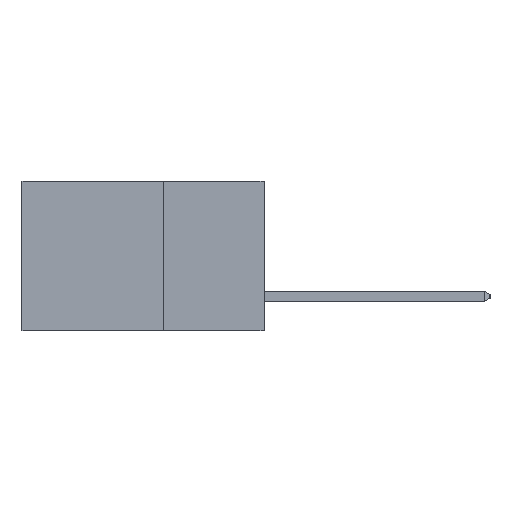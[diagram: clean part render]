
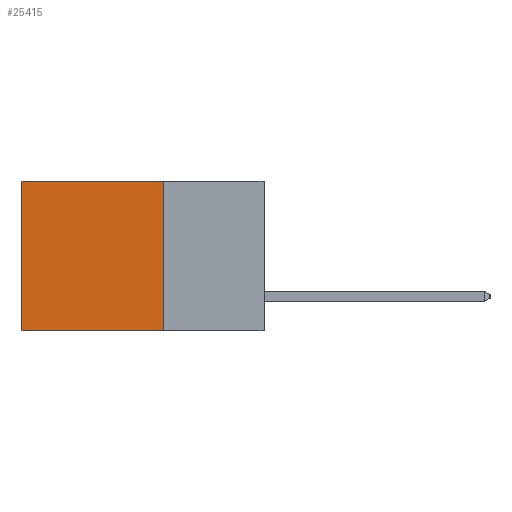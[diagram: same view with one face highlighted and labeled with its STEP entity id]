
A CAD part, left-side view. The second image highlights one B-rep face of the part: STEP entity #25415.
In plain terms, the highlighted planar face has unit normal (-1, 0, 0).
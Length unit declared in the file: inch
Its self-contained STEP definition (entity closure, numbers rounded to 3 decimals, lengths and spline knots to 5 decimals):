
#1158 = EDGE_CURVE ( 'NONE', #21931, #6660, #15601, .T. ) ;
#1533 = CARTESIAN_POINT ( 'NONE',  ( 0.298, 0.25, -0.37 ) ) ;
#1638 = LINE ( 'NONE', #1533, #12215 ) ;
#2496 = CARTESIAN_POINT ( 'NONE',  ( 0.298, 0.25, 0. ) ) ;
#2591 = DIRECTION ( 'NONE',  ( 0., 0., -1. ) ) ;
#2770 = CARTESIAN_POINT ( 'NONE',  ( 0.298, 0.25, 0. ) ) ;
#2794 = DIRECTION ( 'NONE',  ( 0., 0., -1. ) ) ;
#3395 = LINE ( 'NONE', #22034, #25294 ) ;
#3710 = DIRECTION ( 'NONE',  ( 0., 1., 0. ) ) ;
#3746 = ORIENTED_EDGE ( 'NONE', *, *, #8971, .F. ) ;
#4423 = CARTESIAN_POINT ( 'NONE',  ( 0.298, 0.25, -0.37 ) ) ;
#5731 = ORIENTED_EDGE ( 'NONE', *, *, #16220, .T. ) ;
#5945 = VECTOR ( 'NONE', #2794, 39.37008 ) ;
#6660 = VERTEX_POINT ( 'NONE', #10004 ) ;
#7675 = VERTEX_POINT ( 'NONE', #19522 ) ;
#8971 = EDGE_CURVE ( 'NONE', #7675, #15371, #22276, .T. ) ;
#10004 = CARTESIAN_POINT ( 'NONE',  ( 0.298, 0.6, -0.37 ) ) ;
#10329 = EDGE_CURVE ( 'NONE', #15371, #6660, #1638, .T. ) ;
#11084 = CARTESIAN_POINT ( 'NONE',  ( 0.298, 0.6, 0. ) ) ;
#11807 = ORIENTED_EDGE ( 'NONE', *, *, #1158, .T. ) ;
#12215 = VECTOR ( 'NONE', #3710, 39.37008 ) ;
#12715 = FACE_OUTER_BOUND ( 'NONE', #22020, .T. ) ;
#13137 = PLANE ( 'NONE',  #25505 ) ;
#14957 = VECTOR ( 'NONE', #27420, 39.37008 ) ;
#15330 = DIRECTION ( 'NONE',  ( 1., 0., 0. ) ) ;
#15371 = VERTEX_POINT ( 'NONE', #4423 ) ;
#15601 = LINE ( 'NONE', #21620, #14957 ) ;
#15695 = DIRECTION ( 'NONE',  ( 0., 1., 0. ) ) ;
#16220 = EDGE_CURVE ( 'NONE', #7675, #21931, #3395, .T. ) ;
#18146 = ORIENTED_EDGE ( 'NONE', *, *, #10329, .F. ) ;
#19522 = CARTESIAN_POINT ( 'NONE',  ( 0.298, 0.25, 0. ) ) ;
#21620 = CARTESIAN_POINT ( 'NONE',  ( 0.298, 0.6, 0. ) ) ;
#21931 = VERTEX_POINT ( 'NONE', #11084 ) ;
#22020 = EDGE_LOOP ( 'NONE', ( #11807, #18146, #3746, #5731 ) ) ;
#22034 = CARTESIAN_POINT ( 'NONE',  ( 0.298, 0.25, 0. ) ) ;
#22276 = LINE ( 'NONE', #2770, #5945 ) ;
#25294 = VECTOR ( 'NONE', #15695, 39.37008 ) ;
#25415 = ADVANCED_FACE ( 'NONE', ( #12715 ), #13137, .F. ) ;
#25505 = AXIS2_PLACEMENT_3D ( 'NONE', #2496, #15330, #2591 ) ;
#27420 = DIRECTION ( 'NONE',  ( 0., 0., -1. ) ) ;
